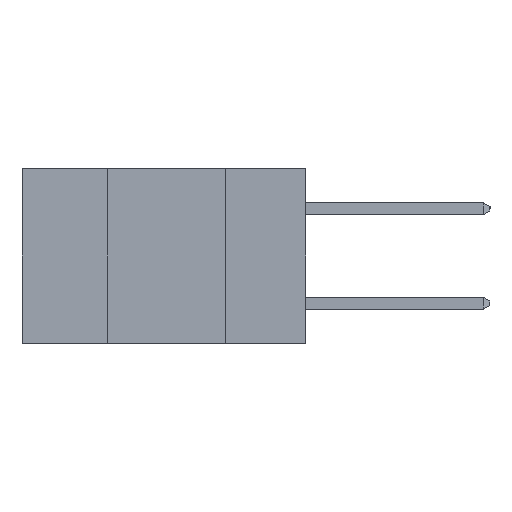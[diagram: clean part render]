
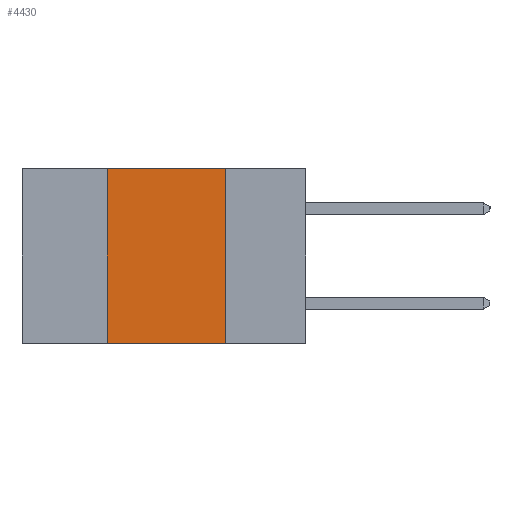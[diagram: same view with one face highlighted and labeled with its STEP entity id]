
A CAD part, left-side view. The second image highlights one B-rep face of the part: STEP entity #4430.
In plain terms, the highlighted planar face has unit normal (-1, 0, 0).
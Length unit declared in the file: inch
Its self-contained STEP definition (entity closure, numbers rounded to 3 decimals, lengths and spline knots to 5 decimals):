
#111 = EDGE_CURVE ( 'NONE', #180, #2556, #8416, .T. ) ;
#180 = VERTEX_POINT ( 'NONE', #1963 ) ;
#661 = LINE ( 'NONE', #4066, #4681 ) ;
#1010 = EDGE_CURVE ( 'NONE', #9795, #2224, #661, .T. ) ;
#1192 = CARTESIAN_POINT ( 'NONE',  ( 0., 0.6, 0. ) ) ;
#1307 = DIRECTION ( 'NONE',  ( 1., 0., 0. ) ) ;
#1478 = EDGE_CURVE ( 'NONE', #180, #9795, #6731, .T. ) ;
#1501 = ORIENTED_EDGE ( 'NONE', *, *, #111, .T. ) ;
#1693 = ORIENTED_EDGE ( 'NONE', *, *, #4352, .F. ) ;
#1963 = CARTESIAN_POINT ( 'NONE',  ( 0., 0.42, -0.37 ) ) ;
#2224 = VERTEX_POINT ( 'NONE', #10131 ) ;
#2556 = VERTEX_POINT ( 'NONE', #6525 ) ;
#2557 = VECTOR ( 'NONE', #10349, 39.37008 ) ;
#2621 = VECTOR ( 'NONE', #7719, 39.37008 ) ;
#3701 = ORIENTED_EDGE ( 'NONE', *, *, #1478, .F. ) ;
#3870 = PLANE ( 'NONE',  #5286 ) ;
#4066 = CARTESIAN_POINT ( 'NONE',  ( 0., 0.6, 0. ) ) ;
#4352 = EDGE_CURVE ( 'NONE', #2224, #2556, #6051, .T. ) ;
#4426 = CARTESIAN_POINT ( 'NONE',  ( 0., 0.17, -0.37 ) ) ;
#4430 = ADVANCED_FACE ( 'NONE', ( #10528 ), #3870, .F. ) ;
#4681 = VECTOR ( 'NONE', #9112, 39.37008 ) ;
#5226 = VECTOR ( 'NONE', #7664, 39.37008 ) ;
#5286 = AXIS2_PLACEMENT_3D ( 'NONE', #1192, #1307, #5406 ) ;
#5406 = DIRECTION ( 'NONE',  ( 0., 0., -1. ) ) ;
#5892 = EDGE_LOOP ( 'NONE', ( #1693, #9626, #3701, #1501 ) ) ;
#6051 = LINE ( 'NONE', #4426, #2621 ) ;
#6525 = CARTESIAN_POINT ( 'NONE',  ( 0., 0.17, -0.37 ) ) ;
#6731 = LINE ( 'NONE', #10151, #5226 ) ;
#7601 = CARTESIAN_POINT ( 'NONE',  ( 0., 0.6, -0.37 ) ) ;
#7664 = DIRECTION ( 'NONE',  ( 0., 0., 1. ) ) ;
#7719 = DIRECTION ( 'NONE',  ( 0., 0., -1. ) ) ;
#7925 = CARTESIAN_POINT ( 'NONE',  ( 0., 0.42, 0. ) ) ;
#8416 = LINE ( 'NONE', #7601, #2557 ) ;
#9112 = DIRECTION ( 'NONE',  ( 0., -1., 0. ) ) ;
#9626 = ORIENTED_EDGE ( 'NONE', *, *, #1010, .F. ) ;
#9795 = VERTEX_POINT ( 'NONE', #7925 ) ;
#10131 = CARTESIAN_POINT ( 'NONE',  ( 0., 0.17, 0. ) ) ;
#10151 = CARTESIAN_POINT ( 'NONE',  ( 0., 0.42, -0.37 ) ) ;
#10349 = DIRECTION ( 'NONE',  ( 0., -1., 0. ) ) ;
#10528 = FACE_OUTER_BOUND ( 'NONE', #5892, .T. ) ;
